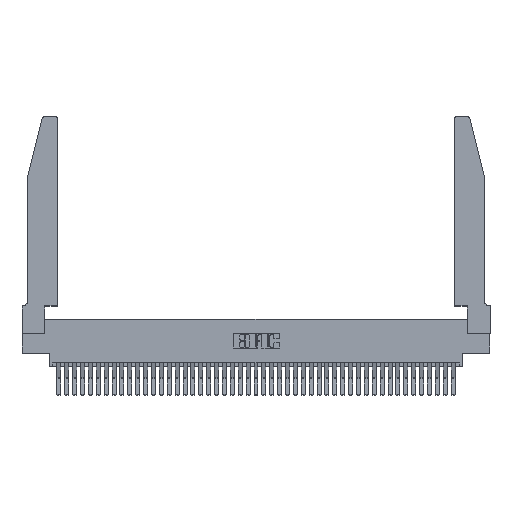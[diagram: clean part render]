
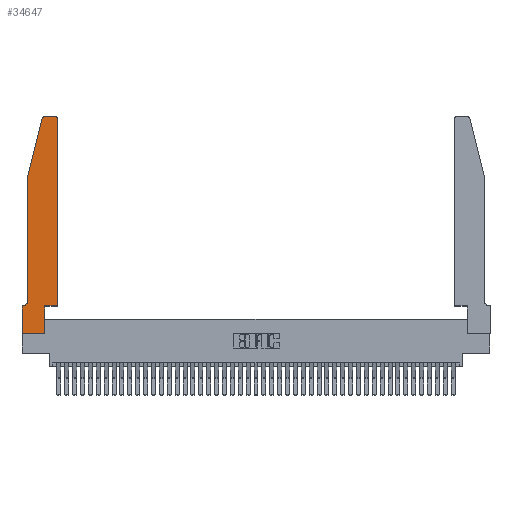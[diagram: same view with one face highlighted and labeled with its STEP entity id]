
A CAD part, top view. The second image highlights one B-rep face of the part: STEP entity #34647.
In plain terms, the highlighted planar face has unit normal (0, 0, 1).
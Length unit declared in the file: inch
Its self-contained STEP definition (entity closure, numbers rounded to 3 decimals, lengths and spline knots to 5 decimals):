
#434 = LINE ( 'NONE', #13410, #34375 ) ;
#450 = DIRECTION ( 'NONE',  ( 0., 0., 1. ) ) ;
#526 = EDGE_CURVE ( 'NONE', #3022, #11020, #23180, .T. ) ;
#1242 = EDGE_CURVE ( 'NONE', #39200, #22267, #28856, .T. ) ;
#1364 = DIRECTION ( 'NONE',  ( 1., 0., 0. ) ) ;
#2089 = LINE ( 'NONE', #11631, #40139 ) ;
#2473 = VERTEX_POINT ( 'NONE', #42789 ) ;
#2642 = FACE_OUTER_BOUND ( 'NONE', #24978, .T. ) ;
#2826 = EDGE_CURVE ( 'NONE', #35338, #2473, #29235, .T. ) ;
#3022 = VERTEX_POINT ( 'NONE', #4000 ) ;
#3847 = VERTEX_POINT ( 'NONE', #19318 ) ;
#4000 = CARTESIAN_POINT ( 'NONE',  ( 0.284, 2.75, 0.37 ) ) ;
#4557 = DIRECTION ( 'NONE',  ( 1., 0., 0. ) ) ;
#4644 = AXIS2_PLACEMENT_3D ( 'NONE', #41860, #26097, #22484 ) ;
#6646 = EDGE_CURVE ( 'NONE', #2473, #39200, #10479, .T. ) ;
#7630 = ORIENTED_EDGE ( 'NONE', *, *, #14112, .T. ) ;
#8088 = ORIENTED_EDGE ( 'NONE', *, *, #32111, .T. ) ;
#8164 = CARTESIAN_POINT ( 'NONE',  ( 0.0055, 0.35, 0.37 ) ) ;
#8827 = CARTESIAN_POINT ( 'NONE',  ( 0., 0.35, 0.37 ) ) ;
#9237 = PLANE ( 'NONE',  #4644 ) ;
#10412 = ORIENTED_EDGE ( 'NONE', *, *, #43776, .T. ) ;
#10479 = LINE ( 'NONE', #25816, #39075 ) ;
#10517 = AXIS2_PLACEMENT_3D ( 'NONE', #30508, #20256, #13974 ) ;
#10889 = VERTEX_POINT ( 'NONE', #33584 ) ;
#11020 = VERTEX_POINT ( 'NONE', #20454 ) ;
#11631 = CARTESIAN_POINT ( 'NONE',  ( 0.4505, 0.35, 0.37 ) ) ;
#12406 = DIRECTION ( 'NONE',  ( 1., 0., 0. ) ) ;
#12642 = DIRECTION ( 'NONE',  ( -0.239, -0.971, 0. ) ) ;
#13008 = CARTESIAN_POINT ( 'NONE',  ( 0.4505, 2.72, 0.37 ) ) ;
#13180 = DIRECTION ( 'NONE',  ( 0., 0., -1. ) ) ;
#13327 = DIRECTION ( 'NONE',  ( -1., 0., 0. ) ) ;
#13410 = CARTESIAN_POINT ( 'NONE',  ( 0.0755, 2., 0.37 ) ) ;
#13974 = DIRECTION ( 'NONE',  ( 1., 0., 0. ) ) ;
#13997 = CIRCLE ( 'NONE', #38566, 0.07 ) ;
#14112 = EDGE_CURVE ( 'NONE', #43548, #10889, #434, .T. ) ;
#14281 = CARTESIAN_POINT ( 'NONE',  ( 0.4505, 0.35, 0.37 ) ) ;
#14457 = CARTESIAN_POINT ( 'NONE',  ( 0.284, 2.72, 0.37 ) ) ;
#14756 = VERTEX_POINT ( 'NONE', #8164 ) ;
#14783 = EDGE_CURVE ( 'NONE', #22267, #43726, #2089, .T. ) ;
#16448 = ORIENTED_EDGE ( 'NONE', *, *, #32499, .T. ) ;
#16738 = CARTESIAN_POINT ( 'NONE',  ( 0.0055, 0.42, 0.37 ) ) ;
#17423 = LINE ( 'NONE', #32828, #39093 ) ;
#18001 = ORIENTED_EDGE ( 'NONE', *, *, #14783, .T. ) ;
#19318 = CARTESIAN_POINT ( 'NONE',  ( 0.4205, 2.75, 0.37 ) ) ;
#20102 = CARTESIAN_POINT ( 'NONE',  ( 0.0755, 2., 0.37 ) ) ;
#20256 = DIRECTION ( 'NONE',  ( 0., 0., 1. ) ) ;
#20382 = CIRCLE ( 'NONE', #10517, 0.03 ) ;
#20454 = CARTESIAN_POINT ( 'NONE',  ( 0.25487, 2.72718, 0.37 ) ) ;
#20512 = DIRECTION ( 'NONE',  ( 0., 1., 0. ) ) ;
#20523 = DIRECTION ( 'NONE',  ( 0., -1., 0. ) ) ;
#21254 = LINE ( 'NONE', #38595, #28654 ) ;
#21531 = DIRECTION ( 'NONE',  ( -1., 0., 0. ) ) ;
#21918 = AXIS2_PLACEMENT_3D ( 'NONE', #14457, #450, #4557 ) ;
#22267 = VERTEX_POINT ( 'NONE', #27837 ) ;
#22484 = DIRECTION ( 'NONE',  ( 1., 0., 0. ) ) ;
#23180 = CIRCLE ( 'NONE', #21918, 0.03 ) ;
#24892 = CARTESIAN_POINT ( 'NONE',  ( 0.2865, 0., 0.37 ) ) ;
#24978 = EDGE_LOOP ( 'NONE', ( #29221, #26693, #28799, #7630, #8088, #33406, #32285, #26793, #30353, #18001, #10412, #16448 ) ) ;
#25311 = EDGE_CURVE ( 'NONE', #3847, #3022, #21254, .T. ) ;
#25816 = CARTESIAN_POINT ( 'NONE',  ( 0., 0., 0.37 ) ) ;
#26097 = DIRECTION ( 'NONE',  ( 0., 0., 1. ) ) ;
#26693 = ORIENTED_EDGE ( 'NONE', *, *, #526, .T. ) ;
#26726 = LINE ( 'NONE', #40337, #31457 ) ;
#26793 = ORIENTED_EDGE ( 'NONE', *, *, #6646, .T. ) ;
#27238 = CARTESIAN_POINT ( 'NONE',  ( 0.4505, 0.35, 0.37 ) ) ;
#27837 = CARTESIAN_POINT ( 'NONE',  ( 0.2865, 0.35, 0.37 ) ) ;
#28654 = VECTOR ( 'NONE', #21531, 39.37008 ) ;
#28799 = ORIENTED_EDGE ( 'NONE', *, *, #42779, .T. ) ;
#28856 = LINE ( 'NONE', #33853, #37288 ) ;
#29221 = ORIENTED_EDGE ( 'NONE', *, *, #25311, .T. ) ;
#29235 = LINE ( 'NONE', #34193, #34488 ) ;
#30353 = ORIENTED_EDGE ( 'NONE', *, *, #1242, .T. ) ;
#30508 = CARTESIAN_POINT ( 'NONE',  ( 0.4205, 2.72, 0.37 ) ) ;
#31457 = VECTOR ( 'NONE', #40475, 39.37008 ) ;
#31569 = EDGE_CURVE ( 'NONE', #14756, #35338, #26726, .T. ) ;
#32111 = EDGE_CURVE ( 'NONE', #10889, #14756, #13997, .T. ) ;
#32285 = ORIENTED_EDGE ( 'NONE', *, *, #2826, .T. ) ;
#32292 = VERTEX_POINT ( 'NONE', #13008 ) ;
#32499 = EDGE_CURVE ( 'NONE', #32292, #3847, #20382, .T. ) ;
#32828 = CARTESIAN_POINT ( 'NONE',  ( 0.0755, 2., 0.37 ) ) ;
#33406 = ORIENTED_EDGE ( 'NONE', *, *, #31569, .T. ) ;
#33584 = CARTESIAN_POINT ( 'NONE',  ( 0.0755, 0.42, 0.37 ) ) ;
#33853 = CARTESIAN_POINT ( 'NONE',  ( 0.2865, 0.35, 0.37 ) ) ;
#34141 = DIRECTION ( 'NONE',  ( 0., 1., 0. ) ) ;
#34193 = CARTESIAN_POINT ( 'NONE',  ( 0., 0., 0.37 ) ) ;
#34375 = VECTOR ( 'NONE', #39959, 39.37008 ) ;
#34488 = VECTOR ( 'NONE', #20523, 39.37008 ) ;
#34647 = ADVANCED_FACE ( 'NONE', ( #2642 ), #9237, .T. ) ;
#35332 = VECTOR ( 'NONE', #20512, 39.37008 ) ;
#35338 = VERTEX_POINT ( 'NONE', #8827 ) ;
#37288 = VECTOR ( 'NONE', #34141, 39.37008 ) ;
#38566 = AXIS2_PLACEMENT_3D ( 'NONE', #16738, #13180, #13327 ) ;
#38595 = CARTESIAN_POINT ( 'NONE',  ( 0.2605, 2.75, 0.37 ) ) ;
#39075 = VECTOR ( 'NONE', #12406, 39.37008 ) ;
#39093 = VECTOR ( 'NONE', #12642, 39.37008 ) ;
#39200 = VERTEX_POINT ( 'NONE', #24892 ) ;
#39959 = DIRECTION ( 'NONE',  ( 0., -1., 0. ) ) ;
#40139 = VECTOR ( 'NONE', #1364, 39.37008 ) ;
#40337 = CARTESIAN_POINT ( 'NONE',  ( 0.0755, 0.35, 0.37 ) ) ;
#40475 = DIRECTION ( 'NONE',  ( -1., 0., 0. ) ) ;
#41860 = CARTESIAN_POINT ( 'NONE',  ( 0., 0.35, 0.37 ) ) ;
#42701 = LINE ( 'NONE', #14281, #35332 ) ;
#42779 = EDGE_CURVE ( 'NONE', #11020, #43548, #17423, .T. ) ;
#42789 = CARTESIAN_POINT ( 'NONE',  ( 0., 0., 0.37 ) ) ;
#43548 = VERTEX_POINT ( 'NONE', #20102 ) ;
#43726 = VERTEX_POINT ( 'NONE', #27238 ) ;
#43776 = EDGE_CURVE ( 'NONE', #43726, #32292, #42701, .T. ) ;
